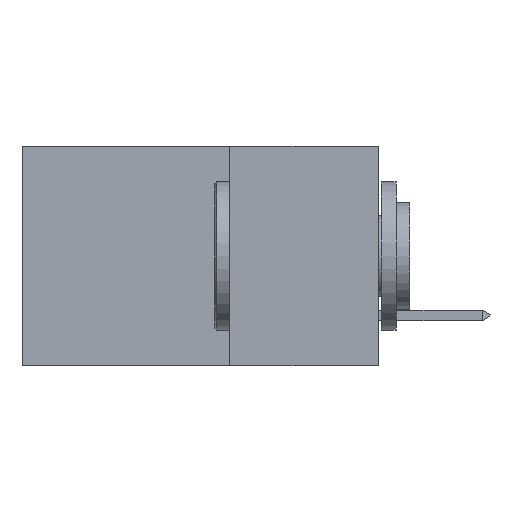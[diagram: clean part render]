
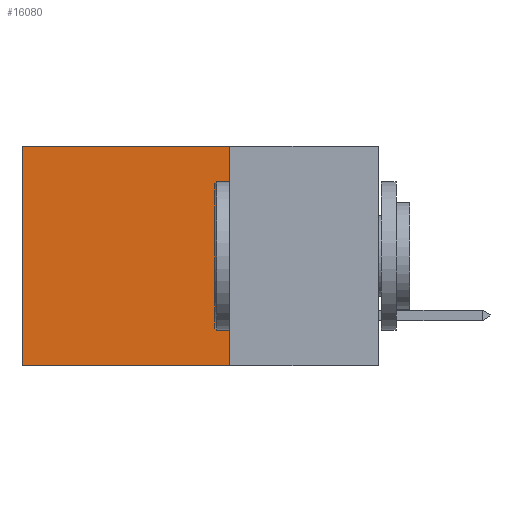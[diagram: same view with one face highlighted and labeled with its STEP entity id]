
A CAD part, left-side view. The second image highlights one B-rep face of the part: STEP entity #16080.
In plain terms, the highlighted planar face has unit normal (-1, 0, 0).
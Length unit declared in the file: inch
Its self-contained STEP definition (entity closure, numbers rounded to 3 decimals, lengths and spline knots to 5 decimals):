
#1964 = ORIENTED_EDGE ( 'NONE', *, *, #9688, .F. ) ;
#2632 = VECTOR ( 'NONE', #11950, 39.37008 ) ;
#2808 = AXIS2_PLACEMENT_3D ( 'NONE', #9238, #4419, #7672 ) ;
#2809 = CARTESIAN_POINT ( 'NONE',  ( 0.2615, 0.25, -0.37 ) ) ;
#3443 = LINE ( 'NONE', #19364, #5289 ) ;
#4419 = DIRECTION ( 'NONE',  ( 1., 0., 0. ) ) ;
#4637 = PLANE ( 'NONE',  #2808 ) ;
#4913 = CARTESIAN_POINT ( 'NONE',  ( 0.2615, 0.6, -0.37 ) ) ;
#5289 = VECTOR ( 'NONE', #13381, 39.37008 ) ;
#5442 = ORIENTED_EDGE ( 'NONE', *, *, #9486, .F. ) ;
#6094 = LINE ( 'NONE', #17310, #16668 ) ;
#6302 = FACE_OUTER_BOUND ( 'NONE', #6941, .T. ) ;
#6941 = EDGE_LOOP ( 'NONE', ( #20241, #5442, #1964, #18584 ) ) ;
#7012 = CARTESIAN_POINT ( 'NONE',  ( 0.2615, 0.25, 0. ) ) ;
#7325 = LINE ( 'NONE', #7012, #14656 ) ;
#7672 = DIRECTION ( 'NONE',  ( 0., 0., -1. ) ) ;
#8071 = EDGE_CURVE ( 'NONE', #18541, #17470, #3443, .T. ) ;
#8591 = EDGE_CURVE ( 'NONE', #12014, #18541, #7325, .T. ) ;
#9238 = CARTESIAN_POINT ( 'NONE',  ( 0.2615, 0.25, -0.37 ) ) ;
#9486 = EDGE_CURVE ( 'NONE', #16513, #17470, #16672, .T. ) ;
#9558 = CARTESIAN_POINT ( 'NONE',  ( 0.2615, 0.25, 0. ) ) ;
#9661 = DIRECTION ( 'NONE',  ( 0., 0., -1. ) ) ;
#9688 = EDGE_CURVE ( 'NONE', #12014, #16513, #6094, .T. ) ;
#10283 = CARTESIAN_POINT ( 'NONE',  ( 0.2615, 0.25, -0.37 ) ) ;
#11950 = DIRECTION ( 'NONE',  ( 0., 1., 0. ) ) ;
#12014 = VERTEX_POINT ( 'NONE', #9558 ) ;
#13215 = CARTESIAN_POINT ( 'NONE',  ( 0.2615, 0.6, 0. ) ) ;
#13381 = DIRECTION ( 'NONE',  ( 0., 0., -1. ) ) ;
#13563 = DIRECTION ( 'NONE',  ( 0., 1., 0. ) ) ;
#14656 = VECTOR ( 'NONE', #13563, 39.37008 ) ;
#16080 = ADVANCED_FACE ( 'NONE', ( #6302 ), #4637, .F. ) ;
#16513 = VERTEX_POINT ( 'NONE', #2809 ) ;
#16668 = VECTOR ( 'NONE', #9661, 39.37008 ) ;
#16672 = LINE ( 'NONE', #10283, #2632 ) ;
#17310 = CARTESIAN_POINT ( 'NONE',  ( 0.2615, 0.25, -0.37 ) ) ;
#17470 = VERTEX_POINT ( 'NONE', #4913 ) ;
#18541 = VERTEX_POINT ( 'NONE', #13215 ) ;
#18584 = ORIENTED_EDGE ( 'NONE', *, *, #8591, .T. ) ;
#19364 = CARTESIAN_POINT ( 'NONE',  ( 0.2615, 0.6, -0.37 ) ) ;
#20241 = ORIENTED_EDGE ( 'NONE', *, *, #8071, .T. ) ;
